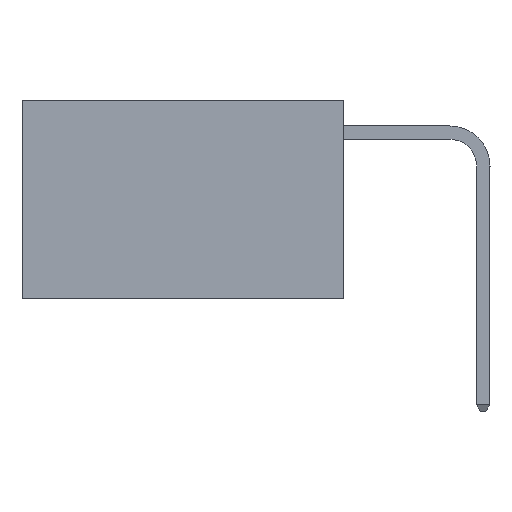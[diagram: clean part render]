
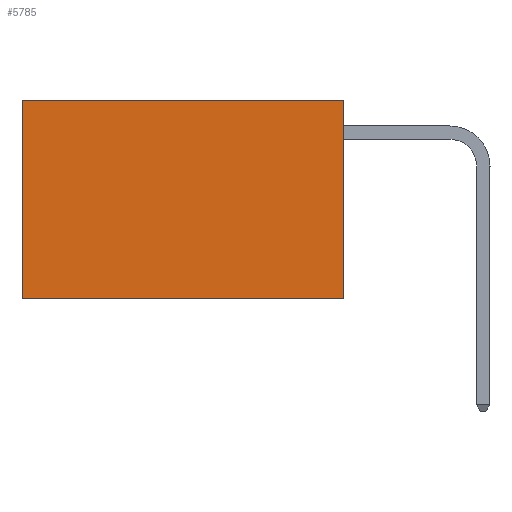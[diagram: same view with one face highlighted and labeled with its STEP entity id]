
A CAD part, left-side view. The second image highlights one B-rep face of the part: STEP entity #5785.
In plain terms, the highlighted planar face has unit normal (-1, 0, 0).
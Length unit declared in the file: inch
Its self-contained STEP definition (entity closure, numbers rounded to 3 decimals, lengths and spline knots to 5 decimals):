
#1187 = VERTEX_POINT ( 'NONE', #4015 ) ;
#1366 = CARTESIAN_POINT ( 'NONE',  ( 0.2625, 0., 0. ) ) ;
#1958 = EDGE_CURVE ( 'NONE', #1187, #11996, #2056, .T. ) ;
#2056 = LINE ( 'NONE', #15466, #11257 ) ;
#4015 = CARTESIAN_POINT ( 'NONE',  ( 0.2625, 0.6, 0. ) ) ;
#4718 = VECTOR ( 'NONE', #5239, 39.37008 ) ;
#5239 = DIRECTION ( 'NONE',  ( 0., 1., 0. ) ) ;
#5754 = VERTEX_POINT ( 'NONE', #21488 ) ;
#5785 = ADVANCED_FACE ( 'NONE', ( #6496 ), #19830, .F. ) ;
#6258 = EDGE_CURVE ( 'NONE', #21003, #5754, #6478, .T. ) ;
#6304 = EDGE_CURVE ( 'NONE', #21003, #1187, #9621, .T. ) ;
#6478 = LINE ( 'NONE', #1366, #15493 ) ;
#6496 = FACE_OUTER_BOUND ( 'NONE', #19349, .T. ) ;
#6946 = DIRECTION ( 'NONE',  ( 0., 0., -1. ) ) ;
#8561 = LINE ( 'NONE', #13595, #12791 ) ;
#9621 = LINE ( 'NONE', #16079, #4718 ) ;
#11257 = VECTOR ( 'NONE', #22643, 39.37008 ) ;
#11996 = VERTEX_POINT ( 'NONE', #15723 ) ;
#12722 = DIRECTION ( 'NONE',  ( 0., 0., -1. ) ) ;
#12791 = VECTOR ( 'NONE', #20776, 39.37008 ) ;
#12809 = ORIENTED_EDGE ( 'NONE', *, *, #6258, .F. ) ;
#13595 = CARTESIAN_POINT ( 'NONE',  ( 0.2625, 0., -0.37 ) ) ;
#14795 = ORIENTED_EDGE ( 'NONE', *, *, #1958, .T. ) ;
#15466 = CARTESIAN_POINT ( 'NONE',  ( 0.2625, 0.6, 0. ) ) ;
#15493 = VECTOR ( 'NONE', #6946, 39.37008 ) ;
#15723 = CARTESIAN_POINT ( 'NONE',  ( 0.2625, 0.6, -0.37 ) ) ;
#16079 = CARTESIAN_POINT ( 'NONE',  ( 0.2625, 0., 0. ) ) ;
#16550 = CARTESIAN_POINT ( 'NONE',  ( 0.2625, 0., 0. ) ) ;
#17216 = ORIENTED_EDGE ( 'NONE', *, *, #18731, .F. ) ;
#17984 = AXIS2_PLACEMENT_3D ( 'NONE', #21639, #23413, #12722 ) ;
#18731 = EDGE_CURVE ( 'NONE', #5754, #11996, #8561, .T. ) ;
#19349 = EDGE_LOOP ( 'NONE', ( #14795, #17216, #12809, #20170 ) ) ;
#19830 = PLANE ( 'NONE',  #17984 ) ;
#20170 = ORIENTED_EDGE ( 'NONE', *, *, #6304, .T. ) ;
#20776 = DIRECTION ( 'NONE',  ( 0., 1., 0. ) ) ;
#21003 = VERTEX_POINT ( 'NONE', #16550 ) ;
#21488 = CARTESIAN_POINT ( 'NONE',  ( 0.2625, 0., -0.37 ) ) ;
#21639 = CARTESIAN_POINT ( 'NONE',  ( 0.2625, 0., 0. ) ) ;
#22643 = DIRECTION ( 'NONE',  ( 0., 0., -1. ) ) ;
#23413 = DIRECTION ( 'NONE',  ( 1., 0., 0. ) ) ;
